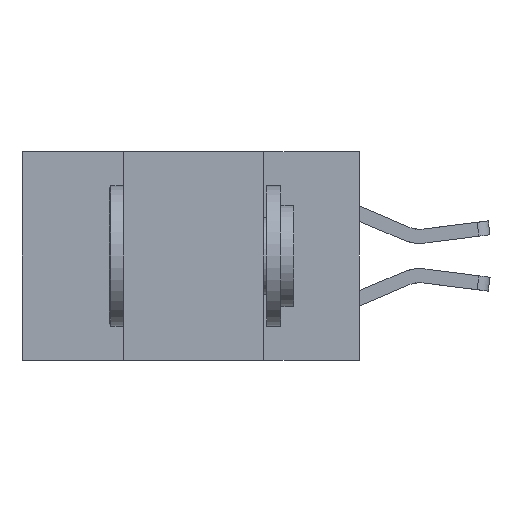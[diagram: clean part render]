
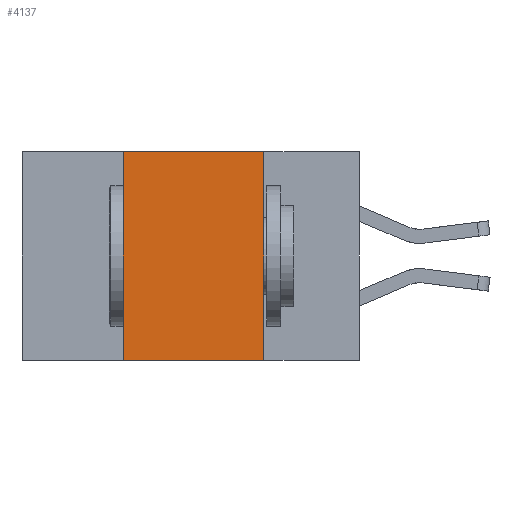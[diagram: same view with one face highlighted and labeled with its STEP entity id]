
A CAD part, left-side view. The second image highlights one B-rep face of the part: STEP entity #4137.
In plain terms, the highlighted planar face has unit normal (-1, 0, 0).
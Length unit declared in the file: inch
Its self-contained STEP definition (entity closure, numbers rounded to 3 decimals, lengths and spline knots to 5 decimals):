
#259 = VECTOR ( 'NONE', #7991, 39.37008 ) ;
#443 = DIRECTION ( 'NONE',  ( 0., 0., -1. ) ) ;
#454 = DIRECTION ( 'NONE',  ( 1., 0., 0. ) ) ;
#518 = CARTESIAN_POINT ( 'NONE',  ( 0., 0.17, 0. ) ) ;
#521 = CARTESIAN_POINT ( 'NONE',  ( 0., 0.6, 0. ) ) ;
#561 = PLANE ( 'NONE',  #8667 ) ;
#1005 = VERTEX_POINT ( 'NONE', #1901 ) ;
#1135 = CARTESIAN_POINT ( 'NONE',  ( 0., 0.17, -0.37 ) ) ;
#1575 = ORIENTED_EDGE ( 'NONE', *, *, #7945, .F. ) ;
#1901 = CARTESIAN_POINT ( 'NONE',  ( 0., 0.42, -0.37 ) ) ;
#2212 = VECTOR ( 'NONE', #3901, 39.37008 ) ;
#2217 = VECTOR ( 'NONE', #5719, 39.37008 ) ;
#2404 = CARTESIAN_POINT ( 'NONE',  ( 0., 0.42, 0. ) ) ;
#2429 = LINE ( 'NONE', #4948, #259 ) ;
#2776 = EDGE_CURVE ( 'NONE', #7421, #4133, #8647, .T. ) ;
#2946 = FACE_OUTER_BOUND ( 'NONE', #5373, .T. ) ;
#3693 = ORIENTED_EDGE ( 'NONE', *, *, #6451, .T. ) ;
#3901 = DIRECTION ( 'NONE',  ( 0., 0., -1. ) ) ;
#4014 = CARTESIAN_POINT ( 'NONE',  ( 0., 0.17, 0. ) ) ;
#4133 = VERTEX_POINT ( 'NONE', #518 ) ;
#4137 = ADVANCED_FACE ( 'NONE', ( #2946 ), #561, .F. ) ;
#4948 = CARTESIAN_POINT ( 'NONE',  ( 0., 0.42, 0. ) ) ;
#5373 = EDGE_LOOP ( 'NONE', ( #5554, #7583, #1575, #3693 ) ) ;
#5554 = ORIENTED_EDGE ( 'NONE', *, *, #6650, .F. ) ;
#5719 = DIRECTION ( 'NONE',  ( 0., -1., 0. ) ) ;
#5817 = LINE ( 'NONE', #6176, #7601 ) ;
#6104 = DIRECTION ( 'NONE',  ( 0., -1., 0. ) ) ;
#6176 = CARTESIAN_POINT ( 'NONE',  ( 0., 0.6, -0.37 ) ) ;
#6451 = EDGE_CURVE ( 'NONE', #1005, #8707, #5817, .T. ) ;
#6453 = CARTESIAN_POINT ( 'NONE',  ( 0., 0.6, 0. ) ) ;
#6650 = EDGE_CURVE ( 'NONE', #4133, #8707, #7937, .T. ) ;
#7421 = VERTEX_POINT ( 'NONE', #2404 ) ;
#7583 = ORIENTED_EDGE ( 'NONE', *, *, #2776, .F. ) ;
#7601 = VECTOR ( 'NONE', #6104, 39.37008 ) ;
#7937 = LINE ( 'NONE', #4014, #2212 ) ;
#7945 = EDGE_CURVE ( 'NONE', #1005, #7421, #2429, .T. ) ;
#7991 = DIRECTION ( 'NONE',  ( 0., 0., 1. ) ) ;
#8647 = LINE ( 'NONE', #6453, #2217 ) ;
#8667 = AXIS2_PLACEMENT_3D ( 'NONE', #521, #454, #443 ) ;
#8707 = VERTEX_POINT ( 'NONE', #1135 ) ;
